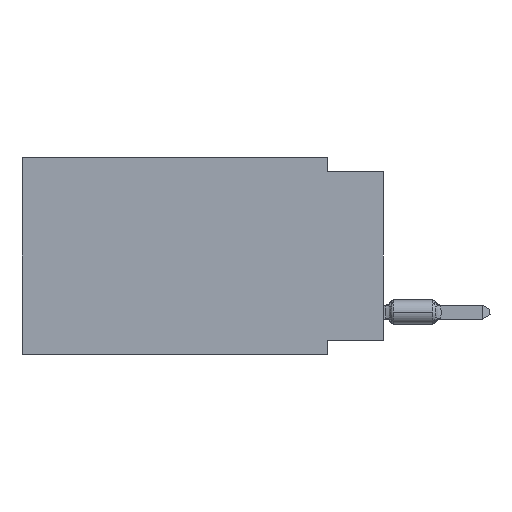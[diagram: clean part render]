
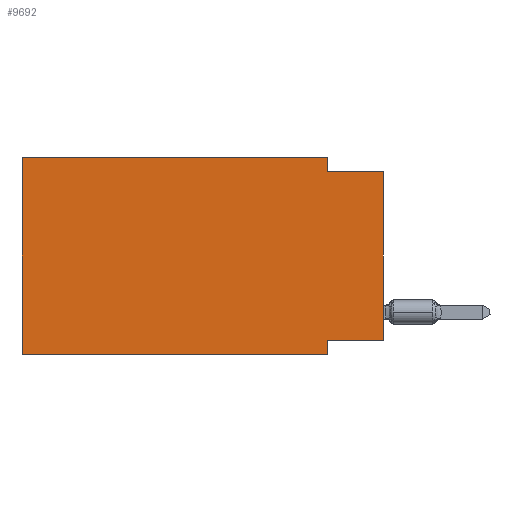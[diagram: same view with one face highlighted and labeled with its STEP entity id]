
A CAD part, left-side view. The second image highlights one B-rep face of the part: STEP entity #9692.
In plain terms, the highlighted planar face has unit normal (-1, 0, 0).
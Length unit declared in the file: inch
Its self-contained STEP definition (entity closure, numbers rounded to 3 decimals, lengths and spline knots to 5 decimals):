
#508 = EDGE_CURVE ( 'NONE', #2998, #13613, #10622, .T. ) ;
#1742 = ORIENTED_EDGE ( 'NONE', *, *, #34250, .F. ) ;
#2506 = LINE ( 'NONE', #28038, #34217 ) ;
#2792 = VECTOR ( 'NONE', #36909, 39.37008 ) ;
#2998 = VERTEX_POINT ( 'NONE', #9437 ) ;
#3373 = LINE ( 'NONE', #17542, #31848 ) ;
#3663 = ORIENTED_EDGE ( 'NONE', *, *, #45875, .F. ) ;
#4720 = FACE_OUTER_BOUND ( 'NONE', #35739, .T. ) ;
#6069 = EDGE_CURVE ( 'NONE', #22807, #9008, #18945, .T. ) ;
#9008 = VERTEX_POINT ( 'NONE', #30155 ) ;
#9437 = CARTESIAN_POINT ( 'NONE',  ( 0., 0.1, 0. ) ) ;
#9692 = ADVANCED_FACE ( 'NONE', ( #4720 ), #14956, .F. ) ;
#10124 = VERTEX_POINT ( 'NONE', #16360 ) ;
#10589 = DIRECTION ( 'NONE',  ( 0., -1., 0. ) ) ;
#10622 = LINE ( 'NONE', #24733, #18947 ) ;
#10849 = DIRECTION ( 'NONE',  ( 0., 1., 0. ) ) ;
#11097 = CARTESIAN_POINT ( 'NONE',  ( 0., 0., -0.025 ) ) ;
#11260 = ORIENTED_EDGE ( 'NONE', *, *, #6069, .F. ) ;
#11933 = DIRECTION ( 'NONE',  ( 1., 0., 0. ) ) ;
#12444 = VECTOR ( 'NONE', #10849, 39.37008 ) ;
#12866 = VECTOR ( 'NONE', #18431, 39.37008 ) ;
#12996 = DIRECTION ( 'NONE',  ( 0., 0., -1. ) ) ;
#13446 = CARTESIAN_POINT ( 'NONE',  ( 0., 0.645, -0.35 ) ) ;
#13613 = VERTEX_POINT ( 'NONE', #19385 ) ;
#14956 = PLANE ( 'NONE',  #33662 ) ;
#15869 = ORIENTED_EDGE ( 'NONE', *, *, #31694, .T. ) ;
#16360 = CARTESIAN_POINT ( 'NONE',  ( 0., 0.1, -0.35 ) ) ;
#16607 = ORIENTED_EDGE ( 'NONE', *, *, #508, .F. ) ;
#17323 = CARTESIAN_POINT ( 'NONE',  ( 0., 0.645, 0. ) ) ;
#17542 = CARTESIAN_POINT ( 'NONE',  ( 0., 0.645, -0.35 ) ) ;
#17998 = LINE ( 'NONE', #17323, #38437 ) ;
#18063 = VERTEX_POINT ( 'NONE', #39237 ) ;
#18431 = DIRECTION ( 'NONE',  ( 0., 0., 1. ) ) ;
#18945 = LINE ( 'NONE', #24959, #12444 ) ;
#18947 = VECTOR ( 'NONE', #21268, 39.37008 ) ;
#19385 = CARTESIAN_POINT ( 'NONE',  ( 0., 0.1, -0.025 ) ) ;
#20825 = LINE ( 'NONE', #42237, #31490 ) ;
#21268 = DIRECTION ( 'NONE',  ( 0., 0., -1. ) ) ;
#22807 = VERTEX_POINT ( 'NONE', #43711 ) ;
#23044 = ORIENTED_EDGE ( 'NONE', *, *, #37790, .T. ) ;
#24113 = EDGE_CURVE ( 'NONE', #38938, #18063, #44777, .T. ) ;
#24733 = CARTESIAN_POINT ( 'NONE',  ( 0., 0.1, 0. ) ) ;
#24959 = CARTESIAN_POINT ( 'NONE',  ( 0., 0., -0.325 ) ) ;
#25265 = VERTEX_POINT ( 'NONE', #11097 ) ;
#25332 = EDGE_CURVE ( 'NONE', #13613, #25265, #20825, .T. ) ;
#26036 = DIRECTION ( 'NONE',  ( 0., 0., -1. ) ) ;
#28038 = CARTESIAN_POINT ( 'NONE',  ( 0., 0.1, -0.35 ) ) ;
#29456 = LINE ( 'NONE', #44128, #2792 ) ;
#30155 = CARTESIAN_POINT ( 'NONE',  ( 0., 0.1, -0.325 ) ) ;
#31490 = VECTOR ( 'NONE', #41991, 39.37008 ) ;
#31694 = EDGE_CURVE ( 'NONE', #22807, #25265, #29456, .T. ) ;
#31848 = VECTOR ( 'NONE', #42417, 39.37008 ) ;
#33662 = AXIS2_PLACEMENT_3D ( 'NONE', #36992, #11933, #26036 ) ;
#34217 = VECTOR ( 'NONE', #12996, 39.37008 ) ;
#34250 = EDGE_CURVE ( 'NONE', #18063, #2998, #17998, .T. ) ;
#35739 = EDGE_LOOP ( 'NONE', ( #15869, #45660, #16607, #1742, #36763, #23044, #3663, #11260 ) ) ;
#36763 = ORIENTED_EDGE ( 'NONE', *, *, #24113, .F. ) ;
#36909 = DIRECTION ( 'NONE',  ( 0., 0., 1. ) ) ;
#36992 = CARTESIAN_POINT ( 'NONE',  ( 0., 0.645, 0. ) ) ;
#37790 = EDGE_CURVE ( 'NONE', #38938, #10124, #3373, .T. ) ;
#38437 = VECTOR ( 'NONE', #10589, 39.37008 ) ;
#38938 = VERTEX_POINT ( 'NONE', #13446 ) ;
#39106 = CARTESIAN_POINT ( 'NONE',  ( 0., 0.645, 0. ) ) ;
#39237 = CARTESIAN_POINT ( 'NONE',  ( 0., 0.645, 0. ) ) ;
#41991 = DIRECTION ( 'NONE',  ( 0., -1., 0. ) ) ;
#42237 = CARTESIAN_POINT ( 'NONE',  ( 0., 0., -0.025 ) ) ;
#42417 = DIRECTION ( 'NONE',  ( 0., -1., 0. ) ) ;
#43711 = CARTESIAN_POINT ( 'NONE',  ( 0., 0., -0.325 ) ) ;
#44128 = CARTESIAN_POINT ( 'NONE',  ( 0., 0., 0. ) ) ;
#44777 = LINE ( 'NONE', #39106, #12866 ) ;
#45660 = ORIENTED_EDGE ( 'NONE', *, *, #25332, .F. ) ;
#45875 = EDGE_CURVE ( 'NONE', #9008, #10124, #2506, .T. ) ;
